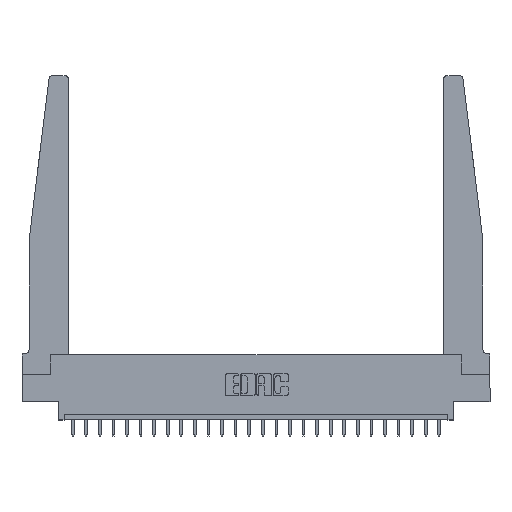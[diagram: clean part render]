
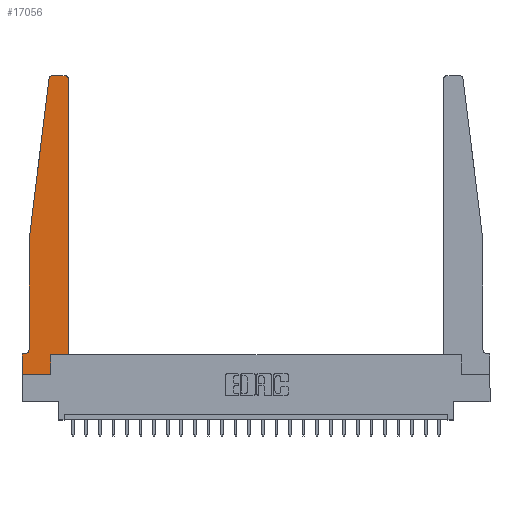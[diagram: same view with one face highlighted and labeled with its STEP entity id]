
A CAD part, top view. The second image highlights one B-rep face of the part: STEP entity #17056.
In plain terms, the highlighted planar face has unit normal (0, 0, 1).
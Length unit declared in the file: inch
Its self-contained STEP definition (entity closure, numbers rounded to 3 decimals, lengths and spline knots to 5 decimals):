
#71 = CARTESIAN_POINT ( 'NONE',  ( 0.065, 1.25, 0.37 ) ) ;
#337 = VECTOR ( 'NONE', #8254, 39.37008 ) ;
#396 = ORIENTED_EDGE ( 'NONE', *, *, #23355, .T. ) ;
#476 = CARTESIAN_POINT ( 'NONE',  ( 0., 0.1875, 0.37 ) ) ;
#1232 = AXIS2_PLACEMENT_3D ( 'NONE', #14472, #12619, #5226 ) ;
#1603 = CARTESIAN_POINT ( 'NONE',  ( 0.065, 0.2375, 0.37 ) ) ;
#2379 = VECTOR ( 'NONE', #17953, 39.37008 ) ;
#2458 = ORIENTED_EDGE ( 'NONE', *, *, #4050, .T. ) ;
#2532 = EDGE_CURVE ( 'NONE', #20077, #10107, #20135, .T. ) ;
#2577 = CIRCLE ( 'NONE', #5621, 0.03 ) ;
#2781 = CARTESIAN_POINT ( 'NONE',  ( 0.25, 2.75, 0.37 ) ) ;
#2836 = DIRECTION ( 'NONE',  ( 1., 0., 0. ) ) ;
#2882 = VERTEX_POINT ( 'NONE', #13475 ) ;
#3023 = LINE ( 'NONE', #11893, #337 ) ;
#3088 = CARTESIAN_POINT ( 'NONE',  ( 0.2605, 0.18, 0.37 ) ) ;
#3158 = CARTESIAN_POINT ( 'NONE',  ( 0.27653, 2.72, 0.37 ) ) ;
#3515 = VERTEX_POINT ( 'NONE', #71 ) ;
#4050 = EDGE_CURVE ( 'NONE', #2882, #20826, #8814, .T. ) ;
#4062 = CARTESIAN_POINT ( 'NONE',  ( 0.425, 0.18, 0.37 ) ) ;
#4201 = ORIENTED_EDGE ( 'NONE', *, *, #20238, .T. ) ;
#4208 = CARTESIAN_POINT ( 'NONE',  ( 0., 0.1875, 0.37 ) ) ;
#4315 = CARTESIAN_POINT ( 'NONE',  ( 0.2605, 0.18, 0.37 ) ) ;
#4686 = VECTOR ( 'NONE', #5201, 39.37008 ) ;
#4694 = FACE_OUTER_BOUND ( 'NONE', #14373, .T. ) ;
#5201 = DIRECTION ( 'NONE',  ( 0., -1., 0. ) ) ;
#5226 = DIRECTION ( 'NONE',  ( -1., 0., 0. ) ) ;
#5248 = VECTOR ( 'NONE', #17647, 39.37008 ) ;
#5402 = VERTEX_POINT ( 'NONE', #24186 ) ;
#5504 = ORIENTED_EDGE ( 'NONE', *, *, #13880, .T. ) ;
#5591 = DIRECTION ( 'NONE',  ( 0., 1., 0. ) ) ;
#5621 = AXIS2_PLACEMENT_3D ( 'NONE', #3158, #23335, #2836 ) ;
#5809 = VECTOR ( 'NONE', #5591, 39.37008 ) ;
#5834 = EDGE_CURVE ( 'NONE', #10368, #14885, #15997, .T. ) ;
#6085 = EDGE_CURVE ( 'NONE', #5402, #2882, #10751, .T. ) ;
#6809 = LINE ( 'NONE', #16447, #17575 ) ;
#7534 = DIRECTION ( 'NONE',  ( 1., 0., 0. ) ) ;
#7846 = DIRECTION ( 'NONE',  ( 1., 0., 0. ) ) ;
#7851 = CARTESIAN_POINT ( 'NONE',  ( 0.395, 2.72, 0.37 ) ) ;
#8254 = DIRECTION ( 'NONE',  ( -0.122, -0.992, 0. ) ) ;
#8297 = CARTESIAN_POINT ( 'NONE',  ( 0., 0., 0.37 ) ) ;
#8320 = ORIENTED_EDGE ( 'NONE', *, *, #20605, .T. ) ;
#8572 = EDGE_CURVE ( 'NONE', #22289, #10368, #20262, .T. ) ;
#8814 = CIRCLE ( 'NONE', #18025, 0.03 ) ;
#9203 = VECTOR ( 'NONE', #13199, 39.37008 ) ;
#9610 = VECTOR ( 'NONE', #16271, 39.37008 ) ;
#9641 = CARTESIAN_POINT ( 'NONE',  ( 0.425, 0.18, 0.37 ) ) ;
#10107 = VERTEX_POINT ( 'NONE', #4315 ) ;
#10146 = ORIENTED_EDGE ( 'NONE', *, *, #5834, .T. ) ;
#10368 = VERTEX_POINT ( 'NONE', #17695 ) ;
#10598 = CARTESIAN_POINT ( 'NONE',  ( 0., 0., 0.37 ) ) ;
#10751 = LINE ( 'NONE', #4062, #5809 ) ;
#11250 = EDGE_CURVE ( 'NONE', #14885, #15966, #13970, .T. ) ;
#11274 = DIRECTION ( 'NONE',  ( 0., 0., 1. ) ) ;
#11893 = CARTESIAN_POINT ( 'NONE',  ( 0.065, 1.25, 0.37 ) ) ;
#11920 = CARTESIAN_POINT ( 'NONE',  ( 0.2605, 0., 0.37 ) ) ;
#12212 = LINE ( 'NONE', #10598, #9610 ) ;
#12402 = DIRECTION ( 'NONE',  ( 0., -1., 0. ) ) ;
#12619 = DIRECTION ( 'NONE',  ( 0., 0., -1. ) ) ;
#12655 = LINE ( 'NONE', #9641, #9203 ) ;
#12831 = CARTESIAN_POINT ( 'NONE',  ( 0., 0., 0.37 ) ) ;
#13199 = DIRECTION ( 'NONE',  ( 1., 0., 0. ) ) ;
#13475 = CARTESIAN_POINT ( 'NONE',  ( 0.425, 2.72, 0.37 ) ) ;
#13675 = DIRECTION ( 'NONE',  ( -1., 0., 0. ) ) ;
#13824 = VERTEX_POINT ( 'NONE', #16144 ) ;
#13880 = EDGE_CURVE ( 'NONE', #10107, #5402, #12655, .T. ) ;
#13970 = LINE ( 'NONE', #12831, #4686 ) ;
#14230 = ORIENTED_EDGE ( 'NONE', *, *, #2532, .T. ) ;
#14373 = EDGE_LOOP ( 'NONE', ( #19861, #15432, #8320, #4201, #22315, #10146, #23515, #396, #14230, #5504, #22601, #2458 ) ) ;
#14472 = CARTESIAN_POINT ( 'NONE',  ( 0.015, 0.2375, 0.37 ) ) ;
#14885 = VERTEX_POINT ( 'NONE', #4208 ) ;
#15432 = ORIENTED_EDGE ( 'NONE', *, *, #18259, .T. ) ;
#15503 = PLANE ( 'NONE',  #19635 ) ;
#15966 = VERTEX_POINT ( 'NONE', #8297 ) ;
#15997 = LINE ( 'NONE', #18985, #17756 ) ;
#16144 = CARTESIAN_POINT ( 'NONE',  ( 0.24675, 2.72367, 0.37 ) ) ;
#16271 = DIRECTION ( 'NONE',  ( 1., 0., 0. ) ) ;
#16447 = CARTESIAN_POINT ( 'NONE',  ( 0.065, 1.25, 0.37 ) ) ;
#16907 = EDGE_CURVE ( 'NONE', #20826, #17107, #21878, .T. ) ;
#17056 = ADVANCED_FACE ( 'NONE', ( #4694 ), #15503, .T. ) ;
#17107 = VERTEX_POINT ( 'NONE', #20784 ) ;
#17575 = VECTOR ( 'NONE', #12402, 39.37008 ) ;
#17647 = DIRECTION ( 'NONE',  ( -1., 0., 0. ) ) ;
#17695 = CARTESIAN_POINT ( 'NONE',  ( 0.015, 0.1875, 0.37 ) ) ;
#17756 = VECTOR ( 'NONE', #13675, 39.37008 ) ;
#17953 = DIRECTION ( 'NONE',  ( 0., 1., 0. ) ) ;
#18025 = AXIS2_PLACEMENT_3D ( 'NONE', #7851, #11274, #7534 ) ;
#18259 = EDGE_CURVE ( 'NONE', #17107, #13824, #2577, .T. ) ;
#18985 = CARTESIAN_POINT ( 'NONE',  ( 0.065, 0.1875, 0.37 ) ) ;
#19635 = AXIS2_PLACEMENT_3D ( 'NONE', #476, #20948, #7846 ) ;
#19861 = ORIENTED_EDGE ( 'NONE', *, *, #16907, .T. ) ;
#20077 = VERTEX_POINT ( 'NONE', #11920 ) ;
#20135 = LINE ( 'NONE', #3088, #2379 ) ;
#20238 = EDGE_CURVE ( 'NONE', #3515, #22289, #6809, .T. ) ;
#20262 = CIRCLE ( 'NONE', #1232, 0.05 ) ;
#20270 = CARTESIAN_POINT ( 'NONE',  ( 0.395, 2.75, 0.37 ) ) ;
#20605 = EDGE_CURVE ( 'NONE', #13824, #3515, #3023, .T. ) ;
#20784 = CARTESIAN_POINT ( 'NONE',  ( 0.27653, 2.75, 0.37 ) ) ;
#20826 = VERTEX_POINT ( 'NONE', #20270 ) ;
#20948 = DIRECTION ( 'NONE',  ( 0., 0., 1. ) ) ;
#21878 = LINE ( 'NONE', #2781, #5248 ) ;
#22289 = VERTEX_POINT ( 'NONE', #1603 ) ;
#22315 = ORIENTED_EDGE ( 'NONE', *, *, #8572, .T. ) ;
#22601 = ORIENTED_EDGE ( 'NONE', *, *, #6085, .T. ) ;
#23335 = DIRECTION ( 'NONE',  ( 0., 0., 1. ) ) ;
#23355 = EDGE_CURVE ( 'NONE', #15966, #20077, #12212, .T. ) ;
#23515 = ORIENTED_EDGE ( 'NONE', *, *, #11250, .T. ) ;
#24186 = CARTESIAN_POINT ( 'NONE',  ( 0.425, 0.18, 0.37 ) ) ;
